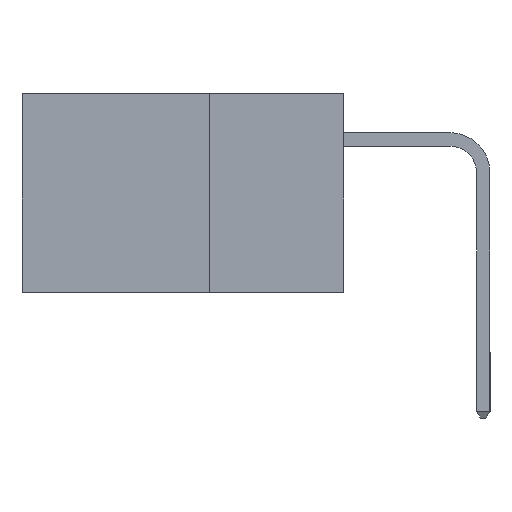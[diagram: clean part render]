
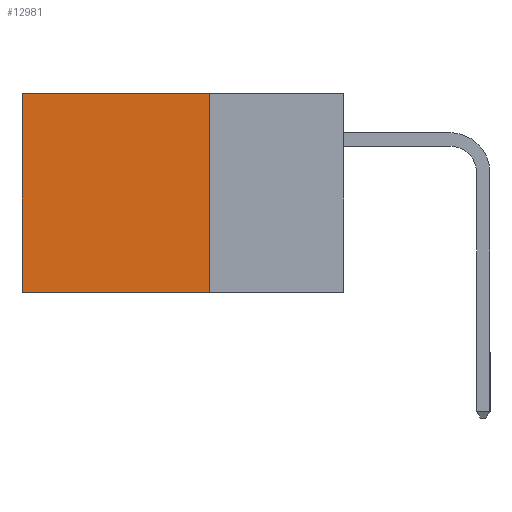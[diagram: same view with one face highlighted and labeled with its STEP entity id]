
A CAD part, left-side view. The second image highlights one B-rep face of the part: STEP entity #12981.
In plain terms, the highlighted planar face has unit normal (-1, 0, 0).
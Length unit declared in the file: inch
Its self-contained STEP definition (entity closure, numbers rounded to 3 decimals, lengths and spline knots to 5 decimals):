
#557 = VERTEX_POINT ( 'NONE', #10081 ) ;
#701 = VERTEX_POINT ( 'NONE', #2748 ) ;
#817 = DIRECTION ( 'NONE',  ( 0., 1., 0. ) ) ;
#1359 = VECTOR ( 'NONE', #8680, 39.37008 ) ;
#1568 = CARTESIAN_POINT ( 'NONE',  ( 0.298, 0.25, 0. ) ) ;
#1909 = CARTESIAN_POINT ( 'NONE',  ( 0.298, 0.25, 0. ) ) ;
#2444 = LINE ( 'NONE', #5482, #12379 ) ;
#2487 = AXIS2_PLACEMENT_3D ( 'NONE', #1568, #5353, #10840 ) ;
#2748 = CARTESIAN_POINT ( 'NONE',  ( 0.298, 0.6, 0. ) ) ;
#3169 = CARTESIAN_POINT ( 'NONE',  ( 0.298, 0.25, -0.37 ) ) ;
#3443 = LINE ( 'NONE', #7447, #9699 ) ;
#3608 = EDGE_CURVE ( 'NONE', #10314, #701, #3443, .T. ) ;
#5070 = ORIENTED_EDGE ( 'NONE', *, *, #12699, .F. ) ;
#5353 = DIRECTION ( 'NONE',  ( 1., 0., 0. ) ) ;
#5482 = CARTESIAN_POINT ( 'NONE',  ( 0.298, 0.6, 0. ) ) ;
#6001 = DIRECTION ( 'NONE',  ( 0., 0., -1. ) ) ;
#6225 = ORIENTED_EDGE ( 'NONE', *, *, #15823, .F. ) ;
#6770 = LINE ( 'NONE', #12522, #1359 ) ;
#6858 = LINE ( 'NONE', #1909, #10177 ) ;
#7447 = CARTESIAN_POINT ( 'NONE',  ( 0.298, 0.25, 0. ) ) ;
#8433 = DIRECTION ( 'NONE',  ( 0., 0., -1. ) ) ;
#8497 = ORIENTED_EDGE ( 'NONE', *, *, #8719, .T. ) ;
#8680 = DIRECTION ( 'NONE',  ( 0., 1., 0. ) ) ;
#8719 = EDGE_CURVE ( 'NONE', #701, #557, #2444, .T. ) ;
#9699 = VECTOR ( 'NONE', #817, 39.37008 ) ;
#10028 = ORIENTED_EDGE ( 'NONE', *, *, #3608, .T. ) ;
#10081 = CARTESIAN_POINT ( 'NONE',  ( 0.298, 0.6, -0.37 ) ) ;
#10177 = VECTOR ( 'NONE', #6001, 39.37008 ) ;
#10314 = VERTEX_POINT ( 'NONE', #16347 ) ;
#10593 = FACE_OUTER_BOUND ( 'NONE', #15718, .T. ) ;
#10840 = DIRECTION ( 'NONE',  ( 0., 0., -1. ) ) ;
#12379 = VECTOR ( 'NONE', #8433, 39.37008 ) ;
#12522 = CARTESIAN_POINT ( 'NONE',  ( 0.298, 0.25, -0.37 ) ) ;
#12699 = EDGE_CURVE ( 'NONE', #10314, #17153, #6858, .T. ) ;
#12981 = ADVANCED_FACE ( 'NONE', ( #10593 ), #14714, .F. ) ;
#14714 = PLANE ( 'NONE',  #2487 ) ;
#15718 = EDGE_LOOP ( 'NONE', ( #8497, #6225, #5070, #10028 ) ) ;
#15823 = EDGE_CURVE ( 'NONE', #17153, #557, #6770, .T. ) ;
#16347 = CARTESIAN_POINT ( 'NONE',  ( 0.298, 0.25, 0. ) ) ;
#17153 = VERTEX_POINT ( 'NONE', #3169 ) ;
